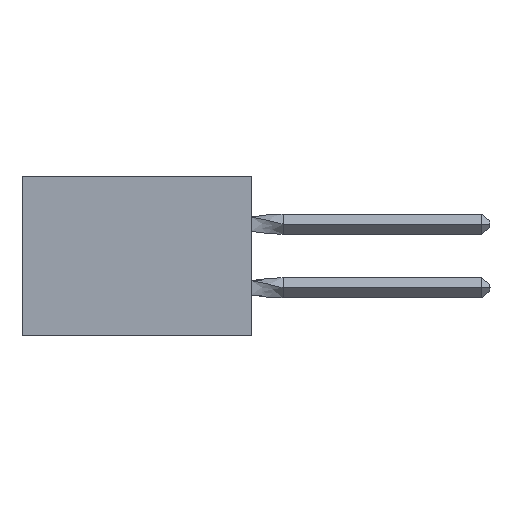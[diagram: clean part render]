
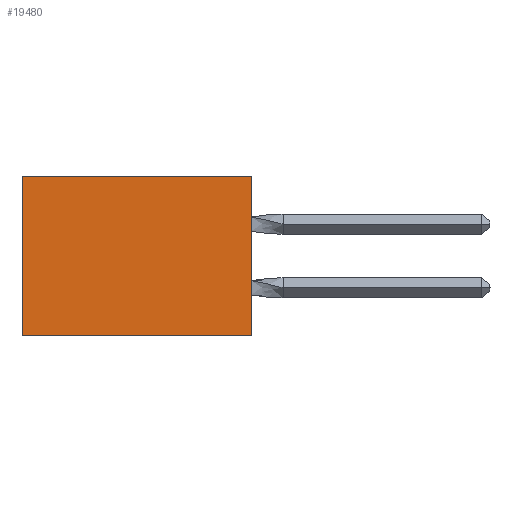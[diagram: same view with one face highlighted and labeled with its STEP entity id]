
A CAD part, left-side view. The second image highlights one B-rep face of the part: STEP entity #19480.
In plain terms, the highlighted planar face has unit normal (-1, 0, 0).
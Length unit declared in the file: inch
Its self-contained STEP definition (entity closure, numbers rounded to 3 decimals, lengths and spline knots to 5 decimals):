
#2723 = DIRECTION ( 'NONE',  ( 0., 1., 0. ) ) ;
#2725 = ORIENTED_EDGE ( 'NONE', *, *, #9479, .T. ) ;
#2813 = LINE ( 'NONE', #23536, #34155 ) ;
#3893 = AXIS2_PLACEMENT_3D ( 'NONE', #23801, #33374, #26881 ) ;
#7631 = VECTOR ( 'NONE', #36505, 39.37008 ) ;
#9431 = CARTESIAN_POINT ( 'NONE',  ( 0.305, 0.72, 0. ) ) ;
#9479 = EDGE_CURVE ( 'NONE', #19197, #13449, #2813, .T. ) ;
#10717 = LINE ( 'NONE', #37925, #32628 ) ;
#11693 = DIRECTION ( 'NONE',  ( 0., 0., -1. ) ) ;
#11958 = ORIENTED_EDGE ( 'NONE', *, *, #34399, .F. ) ;
#13449 = VERTEX_POINT ( 'NONE', #19867 ) ;
#15011 = CARTESIAN_POINT ( 'NONE',  ( 0.305, 0., 0. ) ) ;
#15193 = LINE ( 'NONE', #18419, #7631 ) ;
#18419 = CARTESIAN_POINT ( 'NONE',  ( 0.305, 0., -0.5 ) ) ;
#18985 = CARTESIAN_POINT ( 'NONE',  ( 0.305, 0., -0.5 ) ) ;
#19197 = VERTEX_POINT ( 'NONE', #9431 ) ;
#19480 = ADVANCED_FACE ( 'NONE', ( #35445 ), #20620, .F. ) ;
#19867 = CARTESIAN_POINT ( 'NONE',  ( 0.305, 0.72, -0.5 ) ) ;
#20620 = PLANE ( 'NONE',  #3893 ) ;
#21075 = EDGE_CURVE ( 'NONE', #36447, #19197, #35286, .T. ) ;
#21558 = VERTEX_POINT ( 'NONE', #18985 ) ;
#22956 = ORIENTED_EDGE ( 'NONE', *, *, #36668, .F. ) ;
#23536 = CARTESIAN_POINT ( 'NONE',  ( 0.305, 0.72, -0.5 ) ) ;
#23801 = CARTESIAN_POINT ( 'NONE',  ( 0.305, 0., -0.5 ) ) ;
#24079 = CARTESIAN_POINT ( 'NONE',  ( 0.305, 0., 0. ) ) ;
#25815 = DIRECTION ( 'NONE',  ( 0., 1., 0. ) ) ;
#26632 = ORIENTED_EDGE ( 'NONE', *, *, #21075, .T. ) ;
#26881 = DIRECTION ( 'NONE',  ( 0., 0., -1. ) ) ;
#31013 = VECTOR ( 'NONE', #2723, 39.37008 ) ;
#32628 = VECTOR ( 'NONE', #25815, 39.37008 ) ;
#33374 = DIRECTION ( 'NONE',  ( 1., 0., 0. ) ) ;
#34155 = VECTOR ( 'NONE', #11693, 39.37008 ) ;
#34399 = EDGE_CURVE ( 'NONE', #36447, #21558, #15193, .T. ) ;
#35286 = LINE ( 'NONE', #15011, #31013 ) ;
#35445 = FACE_OUTER_BOUND ( 'NONE', #37224, .T. ) ;
#36447 = VERTEX_POINT ( 'NONE', #24079 ) ;
#36505 = DIRECTION ( 'NONE',  ( 0., 0., -1. ) ) ;
#36668 = EDGE_CURVE ( 'NONE', #21558, #13449, #10717, .T. ) ;
#37224 = EDGE_LOOP ( 'NONE', ( #2725, #22956, #11958, #26632 ) ) ;
#37925 = CARTESIAN_POINT ( 'NONE',  ( 0.305, 0., -0.5 ) ) ;
